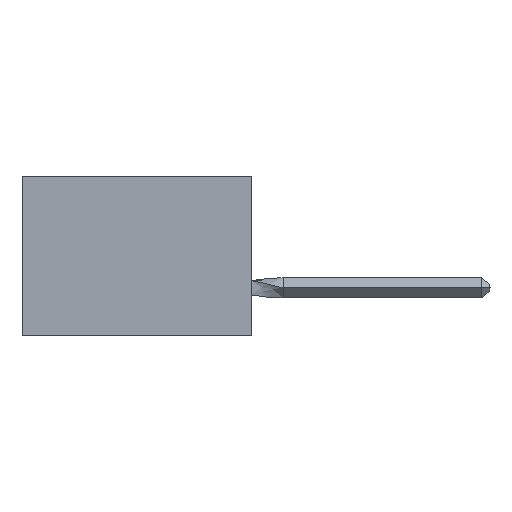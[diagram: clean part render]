
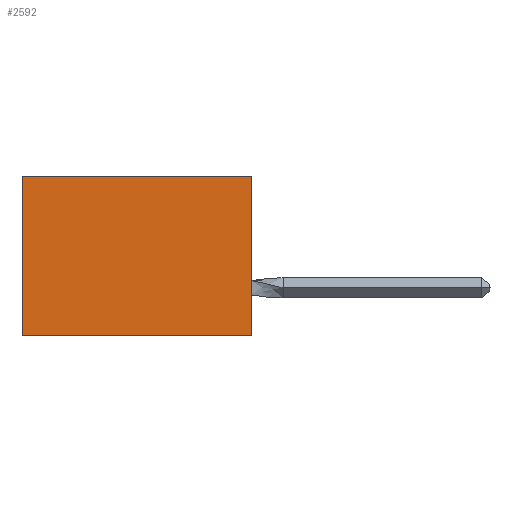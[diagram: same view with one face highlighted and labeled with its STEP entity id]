
A CAD part, left-side view. The second image highlights one B-rep face of the part: STEP entity #2592.
In plain terms, the highlighted planar face has unit normal (-1, 0, 0).
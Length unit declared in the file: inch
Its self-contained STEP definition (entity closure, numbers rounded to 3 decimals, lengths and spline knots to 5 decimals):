
#1321 = CARTESIAN_POINT ( 'NONE',  ( 0.305, 0., 0. ) ) ;
#2494 = EDGE_LOOP ( 'NONE', ( #15875, #6243, #4155, #7714 ) ) ;
#2592 = ADVANCED_FACE ( 'NONE', ( #9520 ), #20851, .F. ) ;
#3109 = CARTESIAN_POINT ( 'NONE',  ( 0.305, 0., -0.5 ) ) ;
#3185 = LINE ( 'NONE', #14446, #12781 ) ;
#4155 = ORIENTED_EDGE ( 'NONE', *, *, #16222, .F. ) ;
#4261 = CARTESIAN_POINT ( 'NONE',  ( 0.305, 0.72, -0.5 ) ) ;
#4567 = DIRECTION ( 'NONE',  ( 0., 0., -1. ) ) ;
#4760 = DIRECTION ( 'NONE',  ( 0., 0., -1. ) ) ;
#4842 = LINE ( 'NONE', #14867, #11915 ) ;
#4871 = CARTESIAN_POINT ( 'NONE',  ( 0.305, 0.72, 0. ) ) ;
#4896 = VERTEX_POINT ( 'NONE', #20044 ) ;
#5499 = DIRECTION ( 'NONE',  ( 0., 0., -1. ) ) ;
#6160 = EDGE_CURVE ( 'NONE', #13469, #16914, #4842, .T. ) ;
#6243 = ORIENTED_EDGE ( 'NONE', *, *, #7312, .F. ) ;
#7010 = VECTOR ( 'NONE', #5499, 39.37008 ) ;
#7312 = EDGE_CURVE ( 'NONE', #4896, #19793, #8584, .T. ) ;
#7714 = ORIENTED_EDGE ( 'NONE', *, *, #6160, .T. ) ;
#8584 = LINE ( 'NONE', #3109, #13635 ) ;
#9495 = DIRECTION ( 'NONE',  ( 1., 0., 0. ) ) ;
#9520 = FACE_OUTER_BOUND ( 'NONE', #2494, .T. ) ;
#9726 = AXIS2_PLACEMENT_3D ( 'NONE', #15937, #9495, #4760 ) ;
#9755 = EDGE_CURVE ( 'NONE', #16914, #19793, #3185, .T. ) ;
#11798 = LINE ( 'NONE', #16942, #7010 ) ;
#11915 = VECTOR ( 'NONE', #18017, 39.37008 ) ;
#12768 = DIRECTION ( 'NONE',  ( 0., 1., 0. ) ) ;
#12781 = VECTOR ( 'NONE', #4567, 39.37008 ) ;
#13469 = VERTEX_POINT ( 'NONE', #1321 ) ;
#13635 = VECTOR ( 'NONE', #12768, 39.37008 ) ;
#14446 = CARTESIAN_POINT ( 'NONE',  ( 0.305, 0.72, -0.5 ) ) ;
#14867 = CARTESIAN_POINT ( 'NONE',  ( 0.305, 0., 0. ) ) ;
#15875 = ORIENTED_EDGE ( 'NONE', *, *, #9755, .T. ) ;
#15937 = CARTESIAN_POINT ( 'NONE',  ( 0.305, 0., -0.5 ) ) ;
#16222 = EDGE_CURVE ( 'NONE', #13469, #4896, #11798, .T. ) ;
#16914 = VERTEX_POINT ( 'NONE', #4871 ) ;
#16942 = CARTESIAN_POINT ( 'NONE',  ( 0.305, 0., -0.5 ) ) ;
#18017 = DIRECTION ( 'NONE',  ( 0., 1., 0. ) ) ;
#19793 = VERTEX_POINT ( 'NONE', #4261 ) ;
#20044 = CARTESIAN_POINT ( 'NONE',  ( 0.305, 0., -0.5 ) ) ;
#20851 = PLANE ( 'NONE',  #9726 ) ;
